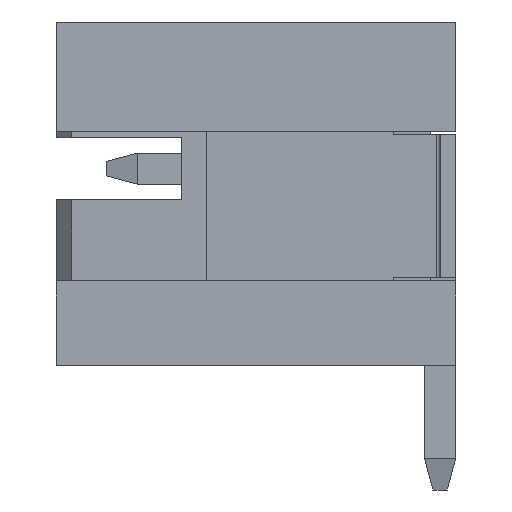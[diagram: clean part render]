
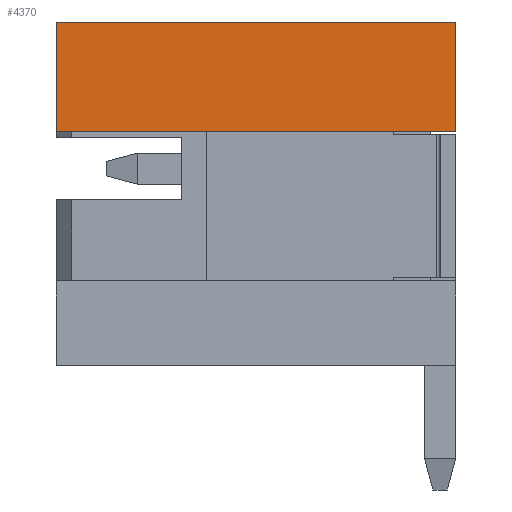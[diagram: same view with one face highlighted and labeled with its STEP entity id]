
A CAD part, left-side view. The second image highlights one B-rep face of the part: STEP entity #4370.
In plain terms, the highlighted planar face has unit normal (-1, 0, 0).
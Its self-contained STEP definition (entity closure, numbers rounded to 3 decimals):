
#147 = LINE ( 'NONE', #2276, #2763 ) ;
#148 = ORIENTED_EDGE ( 'NONE', *, *, #1664, .F. ) ;
#454 = CARTESIAN_POINT ( 'NONE',  ( -3., 6.4, 0.6 ) ) ;
#742 = VECTOR ( 'NONE', #4030, 1000. ) ;
#1012 = LINE ( 'NONE', #5637, #3963 ) ;
#1416 = VERTEX_POINT ( 'NONE', #454 ) ;
#1425 = VERTEX_POINT ( 'NONE', #3459 ) ;
#1607 = PLANE ( 'NONE',  #3021 ) ;
#1661 = ORIENTED_EDGE ( 'NONE', *, *, #5669, .F. ) ;
#1664 = EDGE_CURVE ( 'NONE', #1425, #1416, #4487, .T. ) ;
#1989 = CARTESIAN_POINT ( 'NONE',  ( -3., 0., 0.6 ) ) ;
#1998 = CARTESIAN_POINT ( 'NONE',  ( -3., 0., 2.35 ) ) ;
#2076 = LINE ( 'NONE', #2152, #3742 ) ;
#2118 = DIRECTION ( 'NONE',  ( 1., 0., 0. ) ) ;
#2152 = CARTESIAN_POINT ( 'NONE',  ( -3., 6.4, 2.35 ) ) ;
#2276 = CARTESIAN_POINT ( 'NONE',  ( -3., 0., 2.35 ) ) ;
#2410 = VERTEX_POINT ( 'NONE', #1998 ) ;
#2703 = DIRECTION ( 'NONE',  ( 0., 0., 1. ) ) ;
#2763 = VECTOR ( 'NONE', #5857, 1000. ) ;
#2822 = EDGE_CURVE ( 'NONE', #1416, #4380, #2076, .T. ) ;
#2854 = FACE_OUTER_BOUND ( 'NONE', #6490, .T. ) ;
#3021 = AXIS2_PLACEMENT_3D ( 'NONE', #6160, #2118, #5118 ) ;
#3459 = CARTESIAN_POINT ( 'NONE',  ( -3., 0., 0.6 ) ) ;
#3742 = VECTOR ( 'NONE', #2703, 1000. ) ;
#3963 = VECTOR ( 'NONE', #4290, 1000. ) ;
#4030 = DIRECTION ( 'NONE',  ( 0., 1., 0. ) ) ;
#4114 = CARTESIAN_POINT ( 'NONE',  ( -3., 6.4, 2.35 ) ) ;
#4290 = DIRECTION ( 'NONE',  ( 0., -1., 0. ) ) ;
#4370 = ADVANCED_FACE ( 'NONE', ( #2854 ), #1607, .F. ) ;
#4380 = VERTEX_POINT ( 'NONE', #4114 ) ;
#4487 = LINE ( 'NONE', #1989, #742 ) ;
#4617 = ORIENTED_EDGE ( 'NONE', *, *, #2822, .F. ) ;
#4823 = EDGE_CURVE ( 'NONE', #4380, #2410, #1012, .T. ) ;
#5118 = DIRECTION ( 'NONE',  ( 0., 0., -1. ) ) ;
#5637 = CARTESIAN_POINT ( 'NONE',  ( -3., 6.4, 2.35 ) ) ;
#5669 = EDGE_CURVE ( 'NONE', #2410, #1425, #147, .T. ) ;
#5857 = DIRECTION ( 'NONE',  ( 0., 0., -1. ) ) ;
#6160 = CARTESIAN_POINT ( 'NONE',  ( -3., 0., 0. ) ) ;
#6376 = ORIENTED_EDGE ( 'NONE', *, *, #4823, .F. ) ;
#6490 = EDGE_LOOP ( 'NONE', ( #4617, #148, #1661, #6376 ) ) ;
